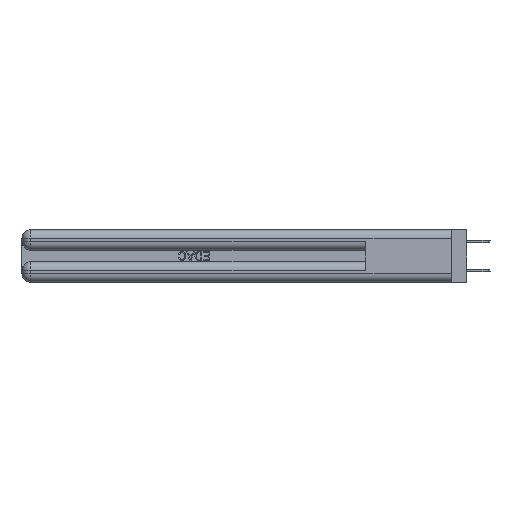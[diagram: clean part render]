
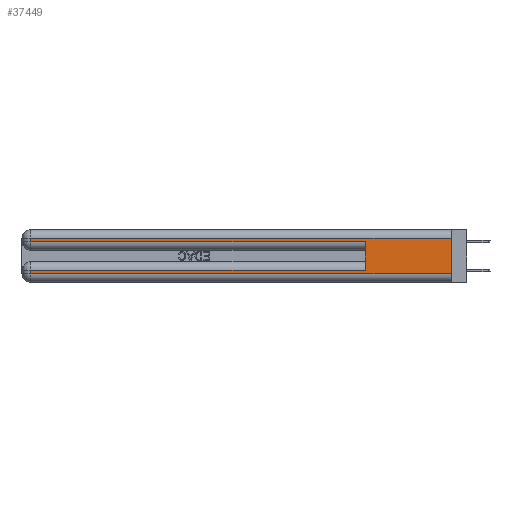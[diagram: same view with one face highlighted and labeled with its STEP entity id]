
A CAD part, left-side view. The second image highlights one B-rep face of the part: STEP entity #37449.
In plain terms, the highlighted planar face has unit normal (-1, 0, 0).
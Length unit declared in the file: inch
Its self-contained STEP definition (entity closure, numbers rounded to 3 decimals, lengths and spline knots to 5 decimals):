
#700 = VERTEX_POINT ( 'NONE', #9862 ) ;
#720 = CARTESIAN_POINT ( 'NONE',  ( 0., 0.6, 0.145 ) ) ;
#730 = AXIS2_PLACEMENT_3D ( 'NONE', #45449, #14267, #13926 ) ;
#1157 = CARTESIAN_POINT ( 'NONE',  ( 0., 0., 0.31 ) ) ;
#3738 = ORIENTED_EDGE ( 'NONE', *, *, #30274, .T. ) ;
#3871 = ORIENTED_EDGE ( 'NONE', *, *, #5551, .T. ) ;
#4824 = DIRECTION ( 'NONE',  ( 0., 0., -1. ) ) ;
#5551 = EDGE_CURVE ( 'NONE', #25407, #9632, #14844, .T. ) ;
#7890 = ORIENTED_EDGE ( 'NONE', *, *, #40554, .T. ) ;
#8174 = LINE ( 'NONE', #720, #22467 ) ;
#8768 = DIRECTION ( 'NONE',  ( 0., 1., 0. ) ) ;
#8859 = VECTOR ( 'NONE', #18039, 39.37008 ) ;
#9632 = VERTEX_POINT ( 'NONE', #10265 ) ;
#9862 = CARTESIAN_POINT ( 'NONE',  ( 0., 2.94, 0.285 ) ) ;
#10265 = CARTESIAN_POINT ( 'NONE',  ( 0., 2.94, 0.085 ) ) ;
#10519 = VECTOR ( 'NONE', #42714, 39.37008 ) ;
#11174 = EDGE_CURVE ( 'NONE', #42695, #15610, #35520, .T. ) ;
#11506 = CARTESIAN_POINT ( 'NONE',  ( 0., 0., 0.06 ) ) ;
#12571 = EDGE_CURVE ( 'NONE', #9632, #42695, #18640, .T. ) ;
#12862 = CARTESIAN_POINT ( 'NONE',  ( 0., 2.94, 0.37 ) ) ;
#13926 = DIRECTION ( 'NONE',  ( 0., 0., -1. ) ) ;
#13979 = CARTESIAN_POINT ( 'NONE',  ( 0., 0.6, 0.085 ) ) ;
#14267 = DIRECTION ( 'NONE',  ( 1., 0., 0. ) ) ;
#14401 = ORIENTED_EDGE ( 'NONE', *, *, #25918, .F. ) ;
#14844 = LINE ( 'NONE', #18342, #10519 ) ;
#15176 = VERTEX_POINT ( 'NONE', #17082 ) ;
#15610 = VERTEX_POINT ( 'NONE', #11506 ) ;
#17082 = CARTESIAN_POINT ( 'NONE',  ( 0., 0., 0.31 ) ) ;
#17904 = DIRECTION ( 'NONE',  ( 0., 0., -1. ) ) ;
#18039 = DIRECTION ( 'NONE',  ( 0., -1., 0. ) ) ;
#18106 = VECTOR ( 'NONE', #8768, 39.37008 ) ;
#18149 = EDGE_LOOP ( 'NONE', ( #14401, #46665, #7890, #3738, #36707, #3871, #35255, #34256 ) ) ;
#18342 = CARTESIAN_POINT ( 'NONE',  ( 0., 0., 0.085 ) ) ;
#18640 = LINE ( 'NONE', #32950, #29854 ) ;
#19890 = DIRECTION ( 'NONE',  ( 0., -1., 0. ) ) ;
#21581 = EDGE_CURVE ( 'NONE', #15176, #45162, #24881, .T. ) ;
#22467 = VECTOR ( 'NONE', #24126, 39.37008 ) ;
#24126 = DIRECTION ( 'NONE',  ( 0., 0., 1. ) ) ;
#24881 = LINE ( 'NONE', #1157, #18106 ) ;
#25407 = VERTEX_POINT ( 'NONE', #13979 ) ;
#25825 = CARTESIAN_POINT ( 'NONE',  ( 0., 0., 0.06 ) ) ;
#25918 = EDGE_CURVE ( 'NONE', #15176, #15610, #26364, .T. ) ;
#26364 = LINE ( 'NONE', #38177, #31917 ) ;
#28051 = CARTESIAN_POINT ( 'NONE',  ( 0., 0., 0.285 ) ) ;
#28813 = LINE ( 'NONE', #12862, #31300 ) ;
#29854 = VECTOR ( 'NONE', #36919, 39.37008 ) ;
#29896 = CARTESIAN_POINT ( 'NONE',  ( 0., 2.94, 0.31 ) ) ;
#30274 = EDGE_CURVE ( 'NONE', #700, #49404, #50605, .T. ) ;
#31300 = VECTOR ( 'NONE', #4824, 39.37008 ) ;
#31917 = VECTOR ( 'NONE', #17904, 39.37008 ) ;
#32950 = CARTESIAN_POINT ( 'NONE',  ( 0., 2.94, 0.37 ) ) ;
#34256 = ORIENTED_EDGE ( 'NONE', *, *, #11174, .T. ) ;
#35255 = ORIENTED_EDGE ( 'NONE', *, *, #12571, .T. ) ;
#35345 = FACE_OUTER_BOUND ( 'NONE', #18149, .T. ) ;
#35520 = LINE ( 'NONE', #25825, #8859 ) ;
#35578 = EDGE_CURVE ( 'NONE', #25407, #49404, #8174, .T. ) ;
#36707 = ORIENTED_EDGE ( 'NONE', *, *, #35578, .F. ) ;
#36919 = DIRECTION ( 'NONE',  ( 0., 0., -1. ) ) ;
#37449 = ADVANCED_FACE ( 'NONE', ( #35345 ), #45796, .F. ) ;
#37559 = VECTOR ( 'NONE', #19890, 39.37008 ) ;
#38177 = CARTESIAN_POINT ( 'NONE',  ( 0., 0., 0.37 ) ) ;
#40554 = EDGE_CURVE ( 'NONE', #45162, #700, #28813, .T. ) ;
#42695 = VERTEX_POINT ( 'NONE', #50618 ) ;
#42714 = DIRECTION ( 'NONE',  ( 0., 1., 0. ) ) ;
#43633 = CARTESIAN_POINT ( 'NONE',  ( 0., 0.6, 0.285 ) ) ;
#45162 = VERTEX_POINT ( 'NONE', #29896 ) ;
#45449 = CARTESIAN_POINT ( 'NONE',  ( 0., 0., 0.37 ) ) ;
#45796 = PLANE ( 'NONE',  #730 ) ;
#46665 = ORIENTED_EDGE ( 'NONE', *, *, #21581, .T. ) ;
#49404 = VERTEX_POINT ( 'NONE', #43633 ) ;
#50605 = LINE ( 'NONE', #28051, #37559 ) ;
#50618 = CARTESIAN_POINT ( 'NONE',  ( 0., 2.94, 0.06 ) ) ;
